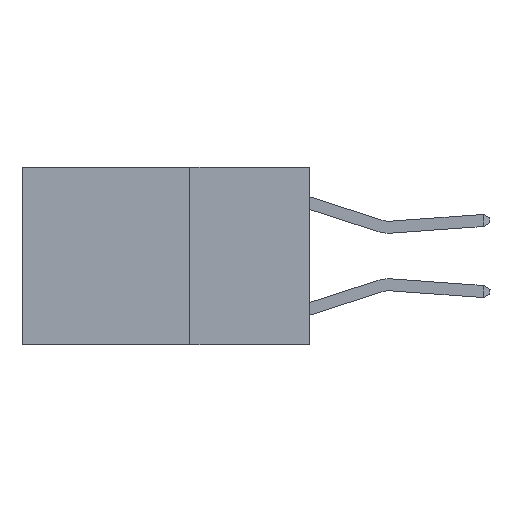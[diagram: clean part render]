
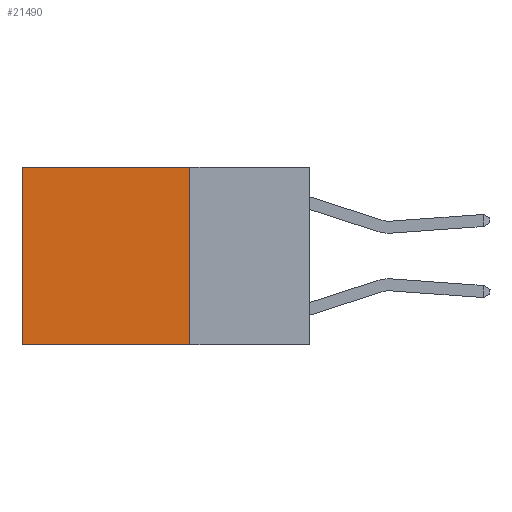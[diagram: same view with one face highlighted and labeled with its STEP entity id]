
A CAD part, left-side view. The second image highlights one B-rep face of the part: STEP entity #21490.
In plain terms, the highlighted planar face has unit normal (-1, 0, 0).
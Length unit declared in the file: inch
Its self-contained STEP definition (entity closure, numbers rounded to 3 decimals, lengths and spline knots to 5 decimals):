
#556 = EDGE_CURVE ( 'NONE', #25414, #11695, #22568, .T. ) ;
#639 = DIRECTION ( 'NONE',  ( 0., 0., -1. ) ) ;
#1914 = CARTESIAN_POINT ( 'NONE',  ( 0.2625, 0.25, -0.37 ) ) ;
#2629 = CARTESIAN_POINT ( 'NONE',  ( 0.2625, 0.6, 0. ) ) ;
#3297 = EDGE_CURVE ( 'NONE', #25414, #16161, #8191, .T. ) ;
#3596 = CARTESIAN_POINT ( 'NONE',  ( 0.2625, 0.25, 0. ) ) ;
#4713 = CARTESIAN_POINT ( 'NONE',  ( 0.2625, 0.25, 0. ) ) ;
#6237 = LINE ( 'NONE', #1914, #11952 ) ;
#7471 = ORIENTED_EDGE ( 'NONE', *, *, #22358, .F. ) ;
#8191 = LINE ( 'NONE', #3596, #9043 ) ;
#9043 = VECTOR ( 'NONE', #25796, 39.37008 ) ;
#9045 = DIRECTION ( 'NONE',  ( 1., 0., 0. ) ) ;
#9354 = EDGE_LOOP ( 'NONE', ( #17460, #7471, #28392, #18890 ) ) ;
#10008 = AXIS2_PLACEMENT_3D ( 'NONE', #18530, #9045, #17830 ) ;
#11695 = VERTEX_POINT ( 'NONE', #24371 ) ;
#11952 = VECTOR ( 'NONE', #15436, 39.37008 ) ;
#13826 = CARTESIAN_POINT ( 'NONE',  ( 0.2625, 0.6, 0. ) ) ;
#15436 = DIRECTION ( 'NONE',  ( 0., 1., 0. ) ) ;
#16161 = VERTEX_POINT ( 'NONE', #2629 ) ;
#17460 = ORIENTED_EDGE ( 'NONE', *, *, #17958, .T. ) ;
#17792 = CARTESIAN_POINT ( 'NONE',  ( 0.2625, 0.25, 0. ) ) ;
#17830 = DIRECTION ( 'NONE',  ( 0., 0., -1. ) ) ;
#17863 = LINE ( 'NONE', #13826, #25563 ) ;
#17958 = EDGE_CURVE ( 'NONE', #16161, #28024, #17863, .T. ) ;
#18010 = DIRECTION ( 'NONE',  ( 0., 0., -1. ) ) ;
#18530 = CARTESIAN_POINT ( 'NONE',  ( 0.2625, 0.25, 0. ) ) ;
#18890 = ORIENTED_EDGE ( 'NONE', *, *, #3297, .T. ) ;
#19548 = PLANE ( 'NONE',  #10008 ) ;
#21490 = ADVANCED_FACE ( 'NONE', ( #24346 ), #19548, .F. ) ;
#22358 = EDGE_CURVE ( 'NONE', #11695, #28024, #6237, .T. ) ;
#22568 = LINE ( 'NONE', #17792, #26586 ) ;
#24346 = FACE_OUTER_BOUND ( 'NONE', #9354, .T. ) ;
#24371 = CARTESIAN_POINT ( 'NONE',  ( 0.2625, 0.25, -0.37 ) ) ;
#25264 = CARTESIAN_POINT ( 'NONE',  ( 0.2625, 0.6, -0.37 ) ) ;
#25414 = VERTEX_POINT ( 'NONE', #4713 ) ;
#25563 = VECTOR ( 'NONE', #18010, 39.37008 ) ;
#25796 = DIRECTION ( 'NONE',  ( 0., 1., 0. ) ) ;
#26586 = VECTOR ( 'NONE', #639, 39.37008 ) ;
#28024 = VERTEX_POINT ( 'NONE', #25264 ) ;
#28392 = ORIENTED_EDGE ( 'NONE', *, *, #556, .F. ) ;
